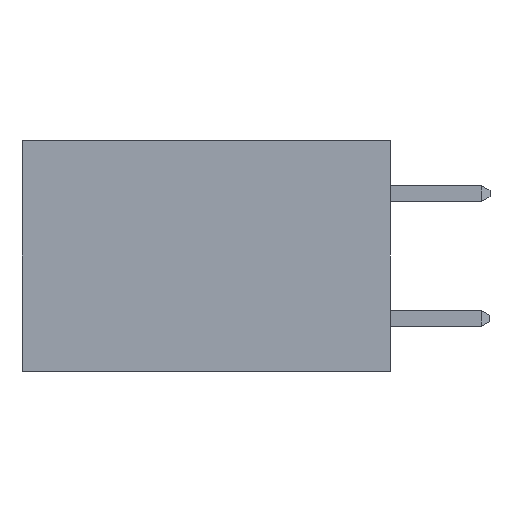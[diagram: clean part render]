
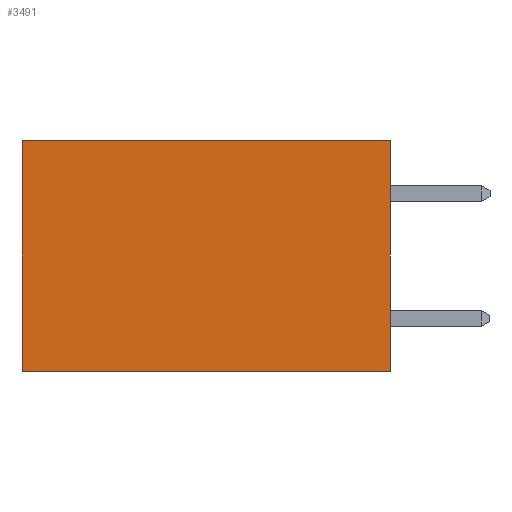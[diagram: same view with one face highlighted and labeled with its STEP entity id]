
A CAD part, left-side view. The second image highlights one B-rep face of the part: STEP entity #3491.
In plain terms, the highlighted planar face has unit normal (-1, 0, 0).
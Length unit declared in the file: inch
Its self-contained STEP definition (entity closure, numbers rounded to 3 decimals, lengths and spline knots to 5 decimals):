
#772 = VERTEX_POINT ( 'NONE', #4060 ) ;
#872 = AXIS2_PLACEMENT_3D ( 'NONE', #2285, #2653, #2255 ) ;
#1055 = LINE ( 'NONE', #7366, #4429 ) ;
#1099 = VERTEX_POINT ( 'NONE', #3574 ) ;
#1540 = DIRECTION ( 'NONE',  ( 0., 1., 0. ) ) ;
#1723 = LINE ( 'NONE', #3676, #7395 ) ;
#1750 = LINE ( 'NONE', #2556, #4752 ) ;
#2255 = DIRECTION ( 'NONE',  ( 0., 0., -1. ) ) ;
#2285 = CARTESIAN_POINT ( 'NONE',  ( 0.277, 0., -0.37 ) ) ;
#2348 = CARTESIAN_POINT ( 'NONE',  ( 0.277, 0.59, 0. ) ) ;
#2358 = PLANE ( 'NONE',  #872 ) ;
#2533 = DIRECTION ( 'NONE',  ( 0., 1., 0. ) ) ;
#2556 = CARTESIAN_POINT ( 'NONE',  ( 0.277, 0., 0. ) ) ;
#2653 = DIRECTION ( 'NONE',  ( 1., 0., 0. ) ) ;
#2676 = ORIENTED_EDGE ( 'NONE', *, *, #3958, .F. ) ;
#2721 = CARTESIAN_POINT ( 'NONE',  ( 0.277, 0., 0. ) ) ;
#3018 = VECTOR ( 'NONE', #3765, 39.37008 ) ;
#3189 = EDGE_CURVE ( 'NONE', #3469, #5032, #1750, .T. ) ;
#3219 = EDGE_CURVE ( 'NONE', #5032, #772, #1055, .T. ) ;
#3469 = VERTEX_POINT ( 'NONE', #2721 ) ;
#3491 = ADVANCED_FACE ( 'NONE', ( #4242 ), #2358, .F. ) ;
#3574 = CARTESIAN_POINT ( 'NONE',  ( 0.277, 0., -0.37 ) ) ;
#3676 = CARTESIAN_POINT ( 'NONE',  ( 0.277, 0., -0.37 ) ) ;
#3765 = DIRECTION ( 'NONE',  ( 0., 0., -1. ) ) ;
#3958 = EDGE_CURVE ( 'NONE', #1099, #772, #1723, .T. ) ;
#4060 = CARTESIAN_POINT ( 'NONE',  ( 0.277, 0.59, -0.37 ) ) ;
#4157 = EDGE_CURVE ( 'NONE', #3469, #1099, #4573, .T. ) ;
#4242 = FACE_OUTER_BOUND ( 'NONE', #4466, .T. ) ;
#4429 = VECTOR ( 'NONE', #7325, 39.37008 ) ;
#4466 = EDGE_LOOP ( 'NONE', ( #6765, #2676, #5686, #6928 ) ) ;
#4573 = LINE ( 'NONE', #5819, #3018 ) ;
#4752 = VECTOR ( 'NONE', #2533, 39.37008 ) ;
#5032 = VERTEX_POINT ( 'NONE', #2348 ) ;
#5686 = ORIENTED_EDGE ( 'NONE', *, *, #4157, .F. ) ;
#5819 = CARTESIAN_POINT ( 'NONE',  ( 0.277, 0., -0.37 ) ) ;
#6765 = ORIENTED_EDGE ( 'NONE', *, *, #3219, .T. ) ;
#6928 = ORIENTED_EDGE ( 'NONE', *, *, #3189, .T. ) ;
#7325 = DIRECTION ( 'NONE',  ( 0., 0., -1. ) ) ;
#7366 = CARTESIAN_POINT ( 'NONE',  ( 0.277, 0.59, -0.37 ) ) ;
#7395 = VECTOR ( 'NONE', #1540, 39.37008 ) ;
